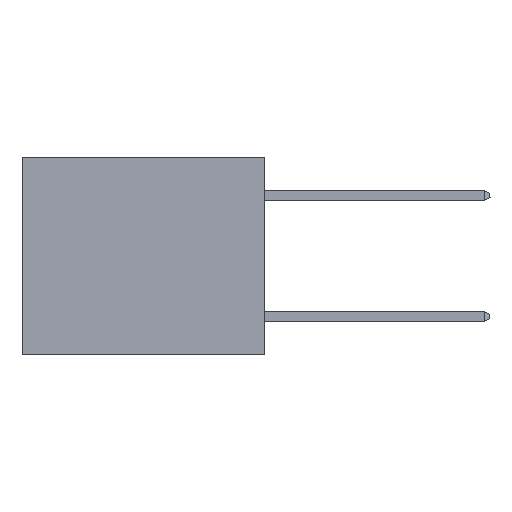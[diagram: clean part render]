
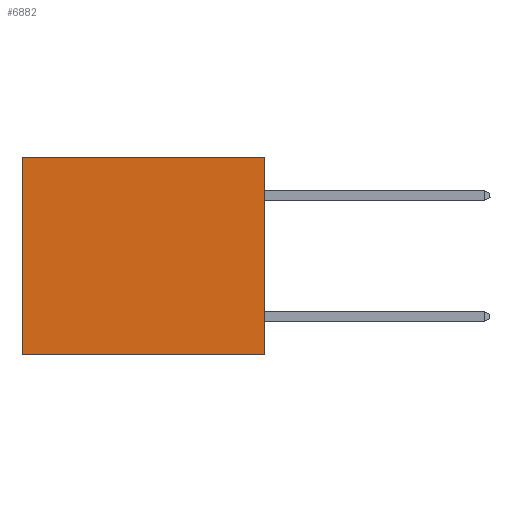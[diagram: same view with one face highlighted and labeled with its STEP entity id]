
A CAD part, left-side view. The second image highlights one B-rep face of the part: STEP entity #6882.
In plain terms, the highlighted planar face has unit normal (-1, 0, 0).
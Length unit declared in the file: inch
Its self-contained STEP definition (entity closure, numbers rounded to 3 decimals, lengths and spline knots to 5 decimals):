
#340 = PLANE ( 'NONE',  #13389 ) ;
#998 = ORIENTED_EDGE ( 'NONE', *, *, #6031, .T. ) ;
#1284 = EDGE_CURVE ( 'NONE', #4283, #18943, #8732, .T. ) ;
#4168 = VECTOR ( 'NONE', #25089, 39.37008 ) ;
#4184 = DIRECTION ( 'NONE',  ( 0., 1., 0. ) ) ;
#4283 = VERTEX_POINT ( 'NONE', #9714 ) ;
#4628 = ORIENTED_EDGE ( 'NONE', *, *, #13825, .T. ) ;
#5005 = LINE ( 'NONE', #6688, #4168 ) ;
#6031 = EDGE_CURVE ( 'NONE', #21501, #18943, #5005, .T. ) ;
#6593 = VECTOR ( 'NONE', #20640, 39.37008 ) ;
#6688 = CARTESIAN_POINT ( 'NONE',  ( 0.3165, 0.6, -0.49 ) ) ;
#6882 = ADVANCED_FACE ( 'NONE', ( #22640 ), #340, .F. ) ;
#7192 = DIRECTION ( 'NONE',  ( 0., 1., 0. ) ) ;
#7826 = LINE ( 'NONE', #13968, #23860 ) ;
#8732 = LINE ( 'NONE', #22909, #16921 ) ;
#9714 = CARTESIAN_POINT ( 'NONE',  ( 0.3165, 0., -0.49 ) ) ;
#10862 = CARTESIAN_POINT ( 'NONE',  ( 0.3165, 0., -0.49 ) ) ;
#11776 = VERTEX_POINT ( 'NONE', #16158 ) ;
#13389 = AXIS2_PLACEMENT_3D ( 'NONE', #10862, #31790, #29264 ) ;
#13555 = EDGE_LOOP ( 'NONE', ( #998, #14986, #25488, #4628 ) ) ;
#13825 = EDGE_CURVE ( 'NONE', #11776, #21501, #7826, .T. ) ;
#13968 = CARTESIAN_POINT ( 'NONE',  ( 0.3165, 0., 0. ) ) ;
#14986 = ORIENTED_EDGE ( 'NONE', *, *, #1284, .F. ) ;
#16158 = CARTESIAN_POINT ( 'NONE',  ( 0.3165, 0., 0. ) ) ;
#16921 = VECTOR ( 'NONE', #7192, 39.37008 ) ;
#18943 = VERTEX_POINT ( 'NONE', #24981 ) ;
#20640 = DIRECTION ( 'NONE',  ( 0., 0., -1. ) ) ;
#21501 = VERTEX_POINT ( 'NONE', #33777 ) ;
#22640 = FACE_OUTER_BOUND ( 'NONE', #13555, .T. ) ;
#22909 = CARTESIAN_POINT ( 'NONE',  ( 0.3165, 0., -0.49 ) ) ;
#23729 = CARTESIAN_POINT ( 'NONE',  ( 0.3165, 0., -0.49 ) ) ;
#23860 = VECTOR ( 'NONE', #4184, 39.37008 ) ;
#24981 = CARTESIAN_POINT ( 'NONE',  ( 0.3165, 0.6, -0.49 ) ) ;
#25089 = DIRECTION ( 'NONE',  ( 0., 0., -1. ) ) ;
#25488 = ORIENTED_EDGE ( 'NONE', *, *, #32174, .F. ) ;
#25548 = LINE ( 'NONE', #23729, #6593 ) ;
#29264 = DIRECTION ( 'NONE',  ( 0., 0., -1. ) ) ;
#31790 = DIRECTION ( 'NONE',  ( 1., 0., 0. ) ) ;
#32174 = EDGE_CURVE ( 'NONE', #11776, #4283, #25548, .T. ) ;
#33777 = CARTESIAN_POINT ( 'NONE',  ( 0.3165, 0.6, 0. ) ) ;
